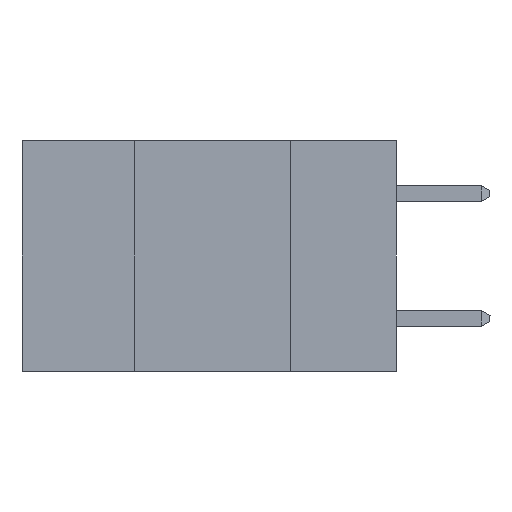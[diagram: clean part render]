
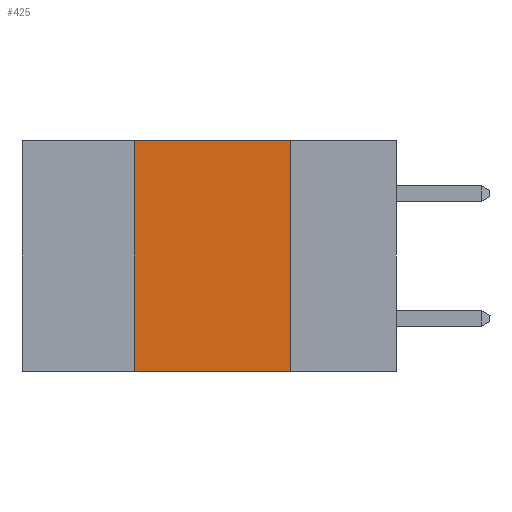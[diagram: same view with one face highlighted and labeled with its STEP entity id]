
A CAD part, left-side view. The second image highlights one B-rep face of the part: STEP entity #425.
In plain terms, the highlighted planar face has unit normal (-1, 0, 0).
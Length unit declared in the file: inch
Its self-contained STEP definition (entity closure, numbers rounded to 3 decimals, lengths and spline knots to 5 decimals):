
#359 = LINE ( 'NONE', #9931, #10643 ) ;
#425 = ADVANCED_FACE ( 'NONE', ( #3123 ), #2733, .F. ) ;
#700 = VERTEX_POINT ( 'NONE', #1630 ) ;
#788 = VERTEX_POINT ( 'NONE', #4746 ) ;
#1226 = ORIENTED_EDGE ( 'NONE', *, *, #3900, .F. ) ;
#1630 = CARTESIAN_POINT ( 'NONE',  ( 0., 0.42, -0.37 ) ) ;
#1944 = EDGE_CURVE ( 'NONE', #700, #6179, #4326, .T. ) ;
#2196 = CARTESIAN_POINT ( 'NONE',  ( 0., 0.42, 0. ) ) ;
#2594 = EDGE_CURVE ( 'NONE', #700, #6542, #4463, .T. ) ;
#2733 = PLANE ( 'NONE',  #11548 ) ;
#3123 = FACE_OUTER_BOUND ( 'NONE', #6015, .T. ) ;
#3358 = CARTESIAN_POINT ( 'NONE',  ( 0., 0.6, 0. ) ) ;
#3501 = ORIENTED_EDGE ( 'NONE', *, *, #5241, .F. ) ;
#3900 = EDGE_CURVE ( 'NONE', #6542, #788, #8517, .T. ) ;
#3980 = DIRECTION ( 'NONE',  ( 1., 0., 0. ) ) ;
#3999 = CARTESIAN_POINT ( 'NONE',  ( 0., 0.6, -0.37 ) ) ;
#4030 = DIRECTION ( 'NONE',  ( 0., -1., 0. ) ) ;
#4326 = LINE ( 'NONE', #3999, #9330 ) ;
#4409 = CARTESIAN_POINT ( 'NONE',  ( 0., 0.17, -0.37 ) ) ;
#4463 = LINE ( 'NONE', #12100, #9473 ) ;
#4547 = DIRECTION ( 'NONE',  ( 0., 0., -1. ) ) ;
#4746 = CARTESIAN_POINT ( 'NONE',  ( 0., 0.17, 0. ) ) ;
#5241 = EDGE_CURVE ( 'NONE', #788, #6179, #359, .T. ) ;
#6015 = EDGE_LOOP ( 'NONE', ( #3501, #1226, #9130, #11785 ) ) ;
#6179 = VERTEX_POINT ( 'NONE', #4409 ) ;
#6542 = VERTEX_POINT ( 'NONE', #2196 ) ;
#6794 = VECTOR ( 'NONE', #11420, 39.37008 ) ;
#8517 = LINE ( 'NONE', #11446, #6794 ) ;
#9130 = ORIENTED_EDGE ( 'NONE', *, *, #2594, .F. ) ;
#9330 = VECTOR ( 'NONE', #4030, 39.37008 ) ;
#9473 = VECTOR ( 'NONE', #11892, 39.37008 ) ;
#9931 = CARTESIAN_POINT ( 'NONE',  ( 0., 0.17, -0.37 ) ) ;
#10054 = DIRECTION ( 'NONE',  ( 0., 0., -1. ) ) ;
#10643 = VECTOR ( 'NONE', #10054, 39.37008 ) ;
#11420 = DIRECTION ( 'NONE',  ( 0., -1., 0. ) ) ;
#11446 = CARTESIAN_POINT ( 'NONE',  ( 0., 0.6, 0. ) ) ;
#11548 = AXIS2_PLACEMENT_3D ( 'NONE', #3358, #3980, #4547 ) ;
#11785 = ORIENTED_EDGE ( 'NONE', *, *, #1944, .T. ) ;
#11892 = DIRECTION ( 'NONE',  ( 0., 0., 1. ) ) ;
#12100 = CARTESIAN_POINT ( 'NONE',  ( 0., 0.42, -0.37 ) ) ;
